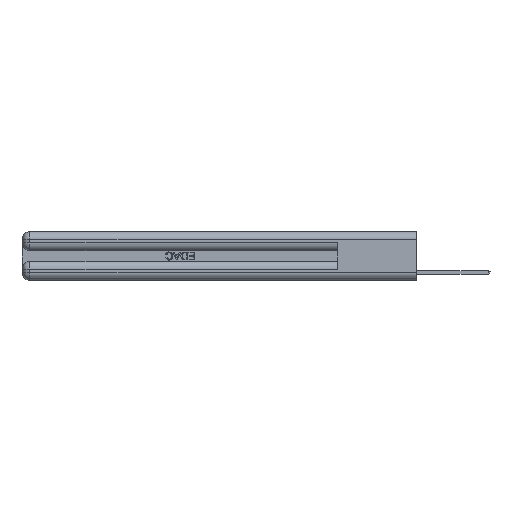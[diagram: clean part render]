
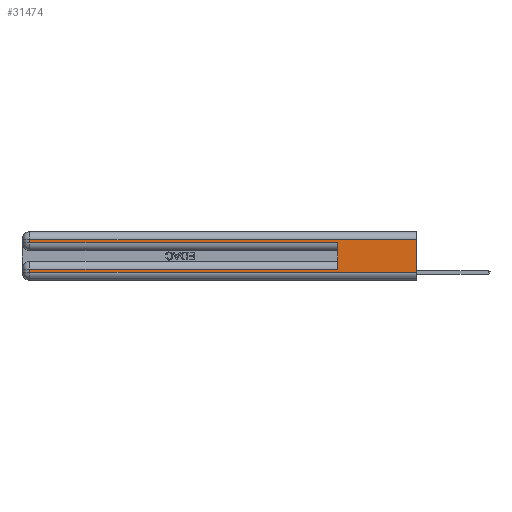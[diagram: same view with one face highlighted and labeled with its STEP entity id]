
A CAD part, left-side view. The second image highlights one B-rep face of the part: STEP entity #31474.
In plain terms, the highlighted planar face has unit normal (-1, 0, 0).
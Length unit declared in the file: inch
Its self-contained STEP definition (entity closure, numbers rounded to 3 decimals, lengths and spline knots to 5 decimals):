
#56 = EDGE_CURVE ( 'NONE', #6228, #30103, #7391, .T. ) ;
#180 = ORIENTED_EDGE ( 'NONE', *, *, #23031, .T. ) ;
#407 = LINE ( 'NONE', #14733, #1551 ) ;
#837 = VERTEX_POINT ( 'NONE', #24914 ) ;
#1311 = LINE ( 'NONE', #16755, #14909 ) ;
#1551 = VECTOR ( 'NONE', #32169, 39.37008 ) ;
#2568 = CARTESIAN_POINT ( 'NONE',  ( 0., 0., 0.085 ) ) ;
#2796 = EDGE_CURVE ( 'NONE', #16753, #12140, #23547, .T. ) ;
#3224 = DIRECTION ( 'NONE',  ( 1., 0., 0. ) ) ;
#4126 = DIRECTION ( 'NONE',  ( 0., 1., 0. ) ) ;
#4340 = VECTOR ( 'NONE', #11193, 39.37008 ) ;
#4868 = CARTESIAN_POINT ( 'NONE',  ( 0., 2.94, 0.37 ) ) ;
#4948 = DIRECTION ( 'NONE',  ( 0., 0., -1. ) ) ;
#6228 = VERTEX_POINT ( 'NONE', #13149 ) ;
#7364 = EDGE_CURVE ( 'NONE', #30593, #6228, #11775, .T. ) ;
#7391 = LINE ( 'NONE', #17340, #15332 ) ;
#7400 = CARTESIAN_POINT ( 'NONE',  ( 0., 2.94, 0.085 ) ) ;
#7640 = LINE ( 'NONE', #4868, #32032 ) ;
#8662 = VERTEX_POINT ( 'NONE', #14230 ) ;
#8812 = ORIENTED_EDGE ( 'NONE', *, *, #17741, .F. ) ;
#8926 = LINE ( 'NONE', #21149, #16391 ) ;
#10770 = ORIENTED_EDGE ( 'NONE', *, *, #11066, .F. ) ;
#11066 = EDGE_CURVE ( 'NONE', #8662, #837, #407, .T. ) ;
#11193 = DIRECTION ( 'NONE',  ( 0., -1., 0. ) ) ;
#11350 = CARTESIAN_POINT ( 'NONE',  ( 0., 0., 0.06 ) ) ;
#11775 = LINE ( 'NONE', #12099, #32193 ) ;
#12099 = CARTESIAN_POINT ( 'NONE',  ( 0., 0., 0.31 ) ) ;
#12140 = VERTEX_POINT ( 'NONE', #28119 ) ;
#12428 = VERTEX_POINT ( 'NONE', #7400 ) ;
#13141 = DIRECTION ( 'NONE',  ( 0., 1., 0. ) ) ;
#13149 = CARTESIAN_POINT ( 'NONE',  ( 0., 2.94, 0.31 ) ) ;
#13155 = DIRECTION ( 'NONE',  ( 0., 0., -1. ) ) ;
#14154 = DIRECTION ( 'NONE',  ( 0., -1., 0. ) ) ;
#14230 = CARTESIAN_POINT ( 'NONE',  ( 0., 0.6, 0.085 ) ) ;
#14733 = CARTESIAN_POINT ( 'NONE',  ( 0., 0.6, 0.145 ) ) ;
#14909 = VECTOR ( 'NONE', #14154, 39.37008 ) ;
#14992 = CARTESIAN_POINT ( 'NONE',  ( 0., 2.94, 0.285 ) ) ;
#15332 = VECTOR ( 'NONE', #4948, 39.37008 ) ;
#16391 = VECTOR ( 'NONE', #28646, 39.37008 ) ;
#16753 = VERTEX_POINT ( 'NONE', #22734 ) ;
#16755 = CARTESIAN_POINT ( 'NONE',  ( 0., 0., 0.285 ) ) ;
#17340 = CARTESIAN_POINT ( 'NONE',  ( 0., 2.94, 0.37 ) ) ;
#17443 = EDGE_CURVE ( 'NONE', #12428, #16753, #7640, .T. ) ;
#17572 = FACE_OUTER_BOUND ( 'NONE', #21765, .T. ) ;
#17741 = EDGE_CURVE ( 'NONE', #30593, #12140, #8926, .T. ) ;
#17811 = AXIS2_PLACEMENT_3D ( 'NONE', #18047, #3224, #13155 ) ;
#18047 = CARTESIAN_POINT ( 'NONE',  ( 0., 0., 0.37 ) ) ;
#21149 = CARTESIAN_POINT ( 'NONE',  ( 0., 0., 0.37 ) ) ;
#21765 = EDGE_LOOP ( 'NONE', ( #8812, #23900, #27684, #180, #10770, #30241, #27636, #31602 ) ) ;
#22734 = CARTESIAN_POINT ( 'NONE',  ( 0., 2.94, 0.06 ) ) ;
#23031 = EDGE_CURVE ( 'NONE', #30103, #837, #1311, .T. ) ;
#23547 = LINE ( 'NONE', #11350, #4340 ) ;
#23900 = ORIENTED_EDGE ( 'NONE', *, *, #7364, .T. ) ;
#24435 = VECTOR ( 'NONE', #13141, 39.37008 ) ;
#24914 = CARTESIAN_POINT ( 'NONE',  ( 0., 0.6, 0.285 ) ) ;
#25347 = LINE ( 'NONE', #2568, #24435 ) ;
#27496 = PLANE ( 'NONE',  #17811 ) ;
#27522 = DIRECTION ( 'NONE',  ( 0., 0., -1. ) ) ;
#27636 = ORIENTED_EDGE ( 'NONE', *, *, #17443, .T. ) ;
#27684 = ORIENTED_EDGE ( 'NONE', *, *, #56, .T. ) ;
#28119 = CARTESIAN_POINT ( 'NONE',  ( 0., 0., 0.06 ) ) ;
#28646 = DIRECTION ( 'NONE',  ( 0., 0., -1. ) ) ;
#28857 = EDGE_CURVE ( 'NONE', #8662, #12428, #25347, .T. ) ;
#30098 = CARTESIAN_POINT ( 'NONE',  ( 0., 0., 0.31 ) ) ;
#30103 = VERTEX_POINT ( 'NONE', #14992 ) ;
#30241 = ORIENTED_EDGE ( 'NONE', *, *, #28857, .T. ) ;
#30593 = VERTEX_POINT ( 'NONE', #30098 ) ;
#31474 = ADVANCED_FACE ( 'NONE', ( #17572 ), #27496, .F. ) ;
#31602 = ORIENTED_EDGE ( 'NONE', *, *, #2796, .T. ) ;
#32032 = VECTOR ( 'NONE', #27522, 39.37008 ) ;
#32169 = DIRECTION ( 'NONE',  ( 0., 0., 1. ) ) ;
#32193 = VECTOR ( 'NONE', #4126, 39.37008 ) ;
